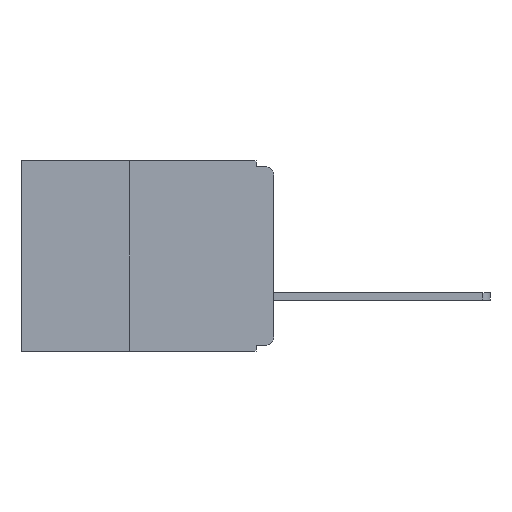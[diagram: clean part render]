
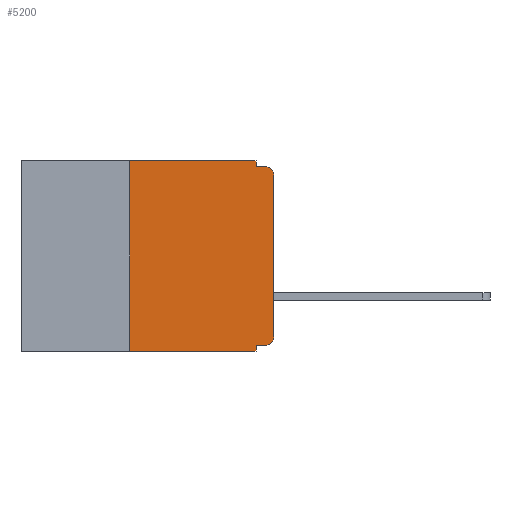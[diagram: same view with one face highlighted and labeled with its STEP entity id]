
A CAD part, left-side view. The second image highlights one B-rep face of the part: STEP entity #5200.
In plain terms, the highlighted planar face has unit normal (-1, 0, 0).
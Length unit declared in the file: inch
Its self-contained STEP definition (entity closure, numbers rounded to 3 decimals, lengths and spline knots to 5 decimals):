
#457 = ORIENTED_EDGE ( 'NONE', *, *, #6014, .T. ) ;
#574 = VERTEX_POINT ( 'NONE', #7627 ) ;
#742 = DIRECTION ( 'NONE',  ( 0., -1., 0. ) ) ;
#959 = VERTEX_POINT ( 'NONE', #12632 ) ;
#982 = EDGE_CURVE ( 'NONE', #12471, #7562, #4468, .T. ) ;
#1362 = AXIS2_PLACEMENT_3D ( 'NONE', #10891, #2395, #12328 ) ;
#1550 = DIRECTION ( 'NONE',  ( 1., 0., 0. ) ) ;
#2275 = ORIENTED_EDGE ( 'NONE', *, *, #982, .F. ) ;
#2395 = DIRECTION ( 'NONE',  ( -1., 0., 0. ) ) ;
#2441 = DIRECTION ( 'NONE',  ( 0., -1., 0. ) ) ;
#3505 = CARTESIAN_POINT ( 'NONE',  ( 0., 0., -0.305 ) ) ;
#4065 = EDGE_LOOP ( 'NONE', ( #457, #15658, #4735, #12721, #16566, #13174, #17020, #2275, #6523, #14100 ) ) ;
#4173 = CIRCLE ( 'NONE', #1362, 0.015 ) ;
#4468 = LINE ( 'NONE', #12755, #11541 ) ;
#4735 = ORIENTED_EDGE ( 'NONE', *, *, #18545, .F. ) ;
#5064 = DIRECTION ( 'NONE',  ( 0., 0., -1. ) ) ;
#5105 = DIRECTION ( 'NONE',  ( -1., 0., 0. ) ) ;
#5167 = CARTESIAN_POINT ( 'NONE',  ( 0., 0.015, -0.025 ) ) ;
#5200 = ADVANCED_FACE ( 'NONE', ( #17461 ), #7384, .F. ) ;
#6014 = EDGE_CURVE ( 'NONE', #7086, #10665, #14064, .T. ) ;
#6160 = DIRECTION ( 'NONE',  ( 0., 0., 1. ) ) ;
#6209 = LINE ( 'NONE', #12720, #13330 ) ;
#6243 = LINE ( 'NONE', #8160, #9567 ) ;
#6451 = VECTOR ( 'NONE', #2441, 39.37008 ) ;
#6523 = ORIENTED_EDGE ( 'NONE', *, *, #10760, .F. ) ;
#6753 = CARTESIAN_POINT ( 'NONE',  ( 0., 0.031, -0.32 ) ) ;
#6878 = VECTOR ( 'NONE', #6160, 39.37008 ) ;
#6932 = VECTOR ( 'NONE', #15450, 39.37008 ) ;
#7086 = VERTEX_POINT ( 'NONE', #3505 ) ;
#7384 = PLANE ( 'NONE',  #8406 ) ;
#7419 = CARTESIAN_POINT ( 'NONE',  ( 0., 0.031, -0.33 ) ) ;
#7444 = VECTOR ( 'NONE', #742, 39.37008 ) ;
#7562 = VERTEX_POINT ( 'NONE', #7419 ) ;
#7627 = CARTESIAN_POINT ( 'NONE',  ( 0., 0.015, -0.01 ) ) ;
#7630 = EDGE_CURVE ( 'NONE', #10665, #574, #12094, .T. ) ;
#8080 = CARTESIAN_POINT ( 'NONE',  ( 0., 0.437, -0.33 ) ) ;
#8160 = CARTESIAN_POINT ( 'NONE',  ( 0., 0.031, 0. ) ) ;
#8173 = VERTEX_POINT ( 'NONE', #13989 ) ;
#8406 = AXIS2_PLACEMENT_3D ( 'NONE', #11178, #1550, #18198 ) ;
#8429 = AXIS2_PLACEMENT_3D ( 'NONE', #5167, #5105, #5064 ) ;
#9567 = VECTOR ( 'NONE', #16752, 39.37008 ) ;
#9710 = EDGE_CURVE ( 'NONE', #8173, #959, #6243, .T. ) ;
#10045 = VERTEX_POINT ( 'NONE', #14688 ) ;
#10191 = LINE ( 'NONE', #8080, #6451 ) ;
#10286 = EDGE_CURVE ( 'NONE', #12337, #7562, #10191, .T. ) ;
#10352 = CARTESIAN_POINT ( 'NONE',  ( 0., 0., -0.025 ) ) ;
#10406 = VERTEX_POINT ( 'NONE', #15535 ) ;
#10608 = DIRECTION ( 'NONE',  ( 0., 1., 0. ) ) ;
#10625 = LINE ( 'NONE', #14739, #6878 ) ;
#10665 = VERTEX_POINT ( 'NONE', #10352 ) ;
#10760 = EDGE_CURVE ( 'NONE', #10045, #12471, #17824, .T. ) ;
#10891 = CARTESIAN_POINT ( 'NONE',  ( 0., 0.015, -0.305 ) ) ;
#11178 = CARTESIAN_POINT ( 'NONE',  ( 0., 0.437, 0. ) ) ;
#11541 = VECTOR ( 'NONE', #14478, 39.37008 ) ;
#12094 = CIRCLE ( 'NONE', #8429, 0.015 ) ;
#12328 = DIRECTION ( 'NONE',  ( 0., 0., -1. ) ) ;
#12337 = VERTEX_POINT ( 'NONE', #13535 ) ;
#12434 = EDGE_CURVE ( 'NONE', #10045, #7086, #4173, .T. ) ;
#12471 = VERTEX_POINT ( 'NONE', #6753 ) ;
#12632 = CARTESIAN_POINT ( 'NONE',  ( 0., 0.031, -0.01 ) ) ;
#12720 = CARTESIAN_POINT ( 'NONE',  ( 0., 0., -0.01 ) ) ;
#12721 = ORIENTED_EDGE ( 'NONE', *, *, #9710, .F. ) ;
#12755 = CARTESIAN_POINT ( 'NONE',  ( 0., 0.031, -0.33 ) ) ;
#12839 = EDGE_CURVE ( 'NONE', #12337, #10406, #10625, .T. ) ;
#13174 = ORIENTED_EDGE ( 'NONE', *, *, #12839, .F. ) ;
#13330 = VECTOR ( 'NONE', #18504, 39.37008 ) ;
#13442 = CARTESIAN_POINT ( 'NONE',  ( 0., 0., -0.32 ) ) ;
#13535 = CARTESIAN_POINT ( 'NONE',  ( 0., 0.25, -0.33 ) ) ;
#13989 = CARTESIAN_POINT ( 'NONE',  ( 0., 0.031, 0. ) ) ;
#14004 = VECTOR ( 'NONE', #10608, 39.37008 ) ;
#14064 = LINE ( 'NONE', #15564, #6932 ) ;
#14100 = ORIENTED_EDGE ( 'NONE', *, *, #12434, .T. ) ;
#14478 = DIRECTION ( 'NONE',  ( 0., 0., -1. ) ) ;
#14688 = CARTESIAN_POINT ( 'NONE',  ( 0., 0.015, -0.32 ) ) ;
#14739 = CARTESIAN_POINT ( 'NONE',  ( 0., 0.25, -0.33 ) ) ;
#14767 = EDGE_CURVE ( 'NONE', #10406, #8173, #15514, .T. ) ;
#14988 = CARTESIAN_POINT ( 'NONE',  ( 0., 0.437, 0. ) ) ;
#15450 = DIRECTION ( 'NONE',  ( 0., 0., 1. ) ) ;
#15514 = LINE ( 'NONE', #14988, #7444 ) ;
#15535 = CARTESIAN_POINT ( 'NONE',  ( 0., 0.25, 0. ) ) ;
#15564 = CARTESIAN_POINT ( 'NONE',  ( 0., 0., 0. ) ) ;
#15658 = ORIENTED_EDGE ( 'NONE', *, *, #7630, .T. ) ;
#16566 = ORIENTED_EDGE ( 'NONE', *, *, #14767, .F. ) ;
#16752 = DIRECTION ( 'NONE',  ( 0., 0., -1. ) ) ;
#17020 = ORIENTED_EDGE ( 'NONE', *, *, #10286, .T. ) ;
#17461 = FACE_OUTER_BOUND ( 'NONE', #4065, .T. ) ;
#17824 = LINE ( 'NONE', #13442, #14004 ) ;
#18198 = DIRECTION ( 'NONE',  ( 0., 0., -1. ) ) ;
#18504 = DIRECTION ( 'NONE',  ( 0., -1., 0. ) ) ;
#18545 = EDGE_CURVE ( 'NONE', #959, #574, #6209, .T. ) ;
